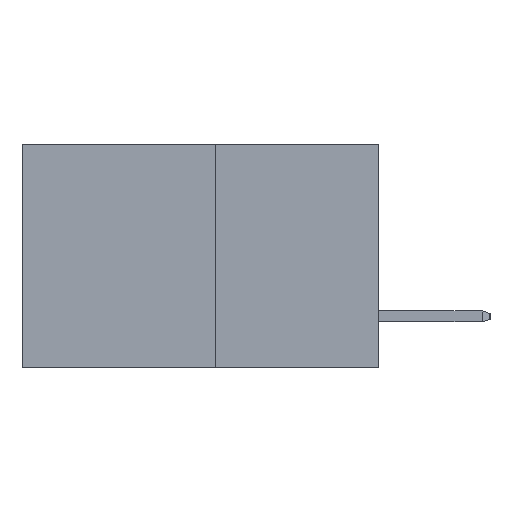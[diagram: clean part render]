
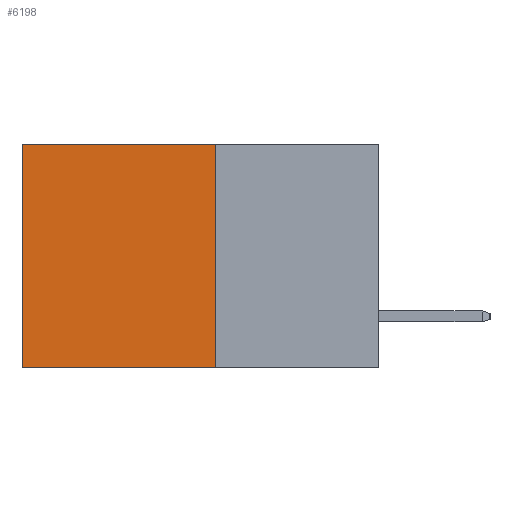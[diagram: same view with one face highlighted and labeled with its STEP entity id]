
A CAD part, left-side view. The second image highlights one B-rep face of the part: STEP entity #6198.
In plain terms, the highlighted planar face has unit normal (-1, 0, 0).
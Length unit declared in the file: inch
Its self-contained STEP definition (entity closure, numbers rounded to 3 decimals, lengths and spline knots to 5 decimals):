
#361 = LINE ( 'NONE', #5024, #2339 ) ;
#2144 = ORIENTED_EDGE ( 'NONE', *, *, #4171, .F. ) ;
#2339 = VECTOR ( 'NONE', #4914, 39.37008 ) ;
#2415 = CARTESIAN_POINT ( 'NONE',  ( 0.277, 0.59, 0. ) ) ;
#2448 = VECTOR ( 'NONE', #12343, 39.37008 ) ;
#2607 = PLANE ( 'NONE',  #11284 ) ;
#2748 = LINE ( 'NONE', #6727, #2448 ) ;
#3379 = VERTEX_POINT ( 'NONE', #2415 ) ;
#3782 = CARTESIAN_POINT ( 'NONE',  ( 0.277, 0.59, -0.37 ) ) ;
#3837 = VECTOR ( 'NONE', #10553, 39.37008 ) ;
#4002 = EDGE_CURVE ( 'NONE', #10384, #11259, #11425, .T. ) ;
#4086 = ORIENTED_EDGE ( 'NONE', *, *, #10474, .T. ) ;
#4128 = CARTESIAN_POINT ( 'NONE',  ( 0.277, 0.27, 0. ) ) ;
#4171 = EDGE_CURVE ( 'NONE', #8873, #10384, #361, .T. ) ;
#4427 = EDGE_LOOP ( 'NONE', ( #4086, #5139, #2144, #9210 ) ) ;
#4523 = DIRECTION ( 'NONE',  ( 1., 0., 0. ) ) ;
#4914 = DIRECTION ( 'NONE',  ( 0., 0., -1. ) ) ;
#5024 = CARTESIAN_POINT ( 'NONE',  ( 0.277, 0.27, -0.37 ) ) ;
#5139 = ORIENTED_EDGE ( 'NONE', *, *, #4002, .F. ) ;
#5568 = CARTESIAN_POINT ( 'NONE',  ( 0.277, 0.27, -0.37 ) ) ;
#6198 = ADVANCED_FACE ( 'NONE', ( #7707 ), #2607, .F. ) ;
#6363 = EDGE_CURVE ( 'NONE', #8873, #3379, #2748, .T. ) ;
#6727 = CARTESIAN_POINT ( 'NONE',  ( 0.277, 0.27, 0. ) ) ;
#7707 = FACE_OUTER_BOUND ( 'NONE', #4427, .T. ) ;
#8617 = VECTOR ( 'NONE', #9530, 39.37008 ) ;
#8873 = VERTEX_POINT ( 'NONE', #4128 ) ;
#9210 = ORIENTED_EDGE ( 'NONE', *, *, #6363, .T. ) ;
#9314 = CARTESIAN_POINT ( 'NONE',  ( 0.277, 0.27, -0.37 ) ) ;
#9530 = DIRECTION ( 'NONE',  ( 0., 0., -1. ) ) ;
#9666 = CARTESIAN_POINT ( 'NONE',  ( 0.277, 0.59, -0.37 ) ) ;
#9905 = LINE ( 'NONE', #3782, #8617 ) ;
#10384 = VERTEX_POINT ( 'NONE', #5568 ) ;
#10474 = EDGE_CURVE ( 'NONE', #3379, #11259, #9905, .T. ) ;
#10553 = DIRECTION ( 'NONE',  ( 0., 1., 0. ) ) ;
#10569 = CARTESIAN_POINT ( 'NONE',  ( 0.277, 0.27, -0.37 ) ) ;
#11173 = DIRECTION ( 'NONE',  ( 0., 0., -1. ) ) ;
#11259 = VERTEX_POINT ( 'NONE', #9666 ) ;
#11284 = AXIS2_PLACEMENT_3D ( 'NONE', #9314, #4523, #11173 ) ;
#11425 = LINE ( 'NONE', #10569, #3837 ) ;
#12343 = DIRECTION ( 'NONE',  ( 0., 1., 0. ) ) ;
